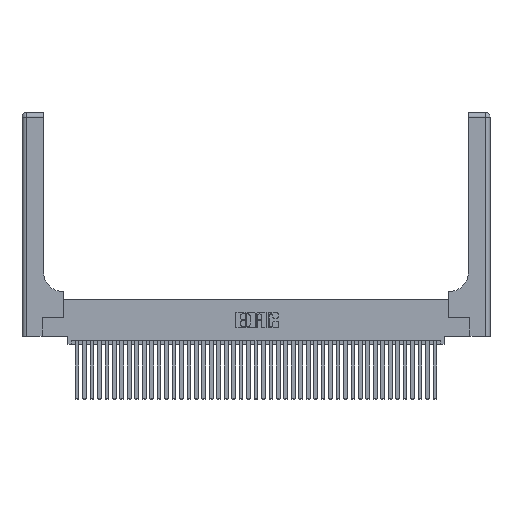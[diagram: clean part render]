
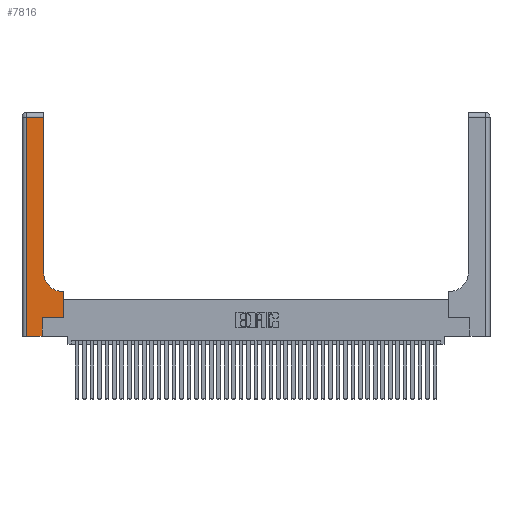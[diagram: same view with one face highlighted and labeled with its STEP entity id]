
A CAD part, top view. The second image highlights one B-rep face of the part: STEP entity #7816.
In plain terms, the highlighted planar face has unit normal (0, 0, 1).
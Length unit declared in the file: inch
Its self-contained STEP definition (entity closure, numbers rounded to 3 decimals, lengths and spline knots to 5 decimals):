
#307 = VECTOR ( 'NONE', #38477, 39.37008 ) ;
#324 = VERTEX_POINT ( 'NONE', #16904 ) ;
#2180 = EDGE_CURVE ( 'NONE', #28909, #26711, #36037, .T. ) ;
#2370 = CARTESIAN_POINT ( 'NONE',  ( 0.5415, 0.6, 0.37 ) ) ;
#2386 = CARTESIAN_POINT ( 'NONE',  ( 0., 2.94, 0.37 ) ) ;
#3132 = CARTESIAN_POINT ( 'NONE',  ( 0., 3., 0.37 ) ) ;
#3900 = ORIENTED_EDGE ( 'NONE', *, *, #6562, .T. ) ;
#5323 = VECTOR ( 'NONE', #35646, 39.37008 ) ;
#6176 = CARTESIAN_POINT ( 'NONE',  ( 0.2915, 0.85, 0.37 ) ) ;
#6255 = CARTESIAN_POINT ( 'NONE',  ( 0.269, 0.25, 0.37 ) ) ;
#6408 = CARTESIAN_POINT ( 'NONE',  ( 0.5585, 0.6, 0.37 ) ) ;
#6562 = EDGE_CURVE ( 'NONE', #38822, #324, #30523, .T. ) ;
#7070 = ORIENTED_EDGE ( 'NONE', *, *, #2180, .T. ) ;
#7729 = ORIENTED_EDGE ( 'NONE', *, *, #9625, .T. ) ;
#7806 = EDGE_LOOP ( 'NONE', ( #8748, #7070, #7729, #3900, #29599, #22634, #14830, #34862, #41850 ) ) ;
#7816 = ADVANCED_FACE ( 'NONE', ( #9331 ), #16210, .F. ) ;
#7882 = DIRECTION ( 'NONE',  ( -1., 0., 0. ) ) ;
#8090 = CARTESIAN_POINT ( 'NONE',  ( 0.5585, 0.25, 0.37 ) ) ;
#8297 = VECTOR ( 'NONE', #26032, 39.37008 ) ;
#8687 = CARTESIAN_POINT ( 'NONE',  ( 0.269, 0., 0.37 ) ) ;
#8748 = ORIENTED_EDGE ( 'NONE', *, *, #40859, .T. ) ;
#9331 = FACE_OUTER_BOUND ( 'NONE', #7806, .T. ) ;
#9625 = EDGE_CURVE ( 'NONE', #26711, #38822, #16080, .T. ) ;
#10989 = VERTEX_POINT ( 'NONE', #2370 ) ;
#11534 = CARTESIAN_POINT ( 'NONE',  ( 0.2915, 2.94, 0.37 ) ) ;
#11695 = VERTEX_POINT ( 'NONE', #15831 ) ;
#12248 = EDGE_CURVE ( 'NONE', #15430, #10989, #12287, .T. ) ;
#12287 = LINE ( 'NONE', #20523, #307 ) ;
#12802 = LINE ( 'NONE', #8687, #36936 ) ;
#14278 = CARTESIAN_POINT ( 'NONE',  ( 0.06, 3., 0.37 ) ) ;
#14830 = ORIENTED_EDGE ( 'NONE', *, *, #18058, .T. ) ;
#15197 = DIRECTION ( 'NONE',  ( 0., 0., -1. ) ) ;
#15430 = VERTEX_POINT ( 'NONE', #6408 ) ;
#15831 = CARTESIAN_POINT ( 'NONE',  ( 0.5585, 0.25, 0.37 ) ) ;
#16080 = LINE ( 'NONE', #14278, #26913 ) ;
#16210 = PLANE ( 'NONE',  #27874 ) ;
#16694 = VERTEX_POINT ( 'NONE', #6176 ) ;
#16904 = CARTESIAN_POINT ( 'NONE',  ( 0.269, 0., 0.37 ) ) ;
#17472 = DIRECTION ( 'NONE',  ( 0., 0., -1. ) ) ;
#18058 = EDGE_CURVE ( 'NONE', #11695, #15430, #18787, .T. ) ;
#18787 = LINE ( 'NONE', #8090, #36753 ) ;
#20258 = EDGE_CURVE ( 'NONE', #10989, #16694, #21233, .T. ) ;
#20523 = CARTESIAN_POINT ( 'NONE',  ( 0.2915, 0.6, 0.37 ) ) ;
#21233 = CIRCLE ( 'NONE', #22353, 0.25 ) ;
#22353 = AXIS2_PLACEMENT_3D ( 'NONE', #28327, #15197, #28626 ) ;
#22634 = ORIENTED_EDGE ( 'NONE', *, *, #34701, .T. ) ;
#23001 = VERTEX_POINT ( 'NONE', #6255 ) ;
#25451 = VECTOR ( 'NONE', #28967, 39.37008 ) ;
#25667 = CARTESIAN_POINT ( 'NONE',  ( 0.269, 0.25, 0.37 ) ) ;
#25968 = LINE ( 'NONE', #42429, #5323 ) ;
#26032 = DIRECTION ( 'NONE',  ( -1., 0., 0. ) ) ;
#26711 = VERTEX_POINT ( 'NONE', #30652 ) ;
#26913 = VECTOR ( 'NONE', #34570, 39.37008 ) ;
#27874 = AXIS2_PLACEMENT_3D ( 'NONE', #3132, #17472, #7882 ) ;
#28327 = CARTESIAN_POINT ( 'NONE',  ( 0.5415, 0.85, 0.37 ) ) ;
#28626 = DIRECTION ( 'NONE',  ( 1., 0., 0. ) ) ;
#28685 = DIRECTION ( 'NONE',  ( 0., 1., 0. ) ) ;
#28909 = VERTEX_POINT ( 'NONE', #11534 ) ;
#28967 = DIRECTION ( 'NONE',  ( 1., 0., 0. ) ) ;
#29532 = VECTOR ( 'NONE', #38894, 39.37008 ) ;
#29599 = ORIENTED_EDGE ( 'NONE', *, *, #38305, .T. ) ;
#30523 = LINE ( 'NONE', #38464, #29532 ) ;
#30652 = CARTESIAN_POINT ( 'NONE',  ( 0.06, 2.94, 0.37 ) ) ;
#31610 = CARTESIAN_POINT ( 'NONE',  ( 0.06, 0., 0.37 ) ) ;
#34570 = DIRECTION ( 'NONE',  ( 0., -1., 0. ) ) ;
#34701 = EDGE_CURVE ( 'NONE', #23001, #11695, #35663, .T. ) ;
#34862 = ORIENTED_EDGE ( 'NONE', *, *, #12248, .T. ) ;
#35646 = DIRECTION ( 'NONE',  ( 0., 1., 0. ) ) ;
#35663 = LINE ( 'NONE', #25667, #25451 ) ;
#36037 = LINE ( 'NONE', #2386, #8297 ) ;
#36753 = VECTOR ( 'NONE', #37701, 39.37008 ) ;
#36936 = VECTOR ( 'NONE', #28685, 39.37008 ) ;
#37701 = DIRECTION ( 'NONE',  ( 0., 1., 0. ) ) ;
#38305 = EDGE_CURVE ( 'NONE', #324, #23001, #12802, .T. ) ;
#38464 = CARTESIAN_POINT ( 'NONE',  ( 0., 0., 0.37 ) ) ;
#38477 = DIRECTION ( 'NONE',  ( -1., 0., 0. ) ) ;
#38822 = VERTEX_POINT ( 'NONE', #31610 ) ;
#38894 = DIRECTION ( 'NONE',  ( 1., 0., 0. ) ) ;
#40859 = EDGE_CURVE ( 'NONE', #16694, #28909, #25968, .T. ) ;
#41850 = ORIENTED_EDGE ( 'NONE', *, *, #20258, .T. ) ;
#42429 = CARTESIAN_POINT ( 'NONE',  ( 0.2915, 3., 0.37 ) ) ;
